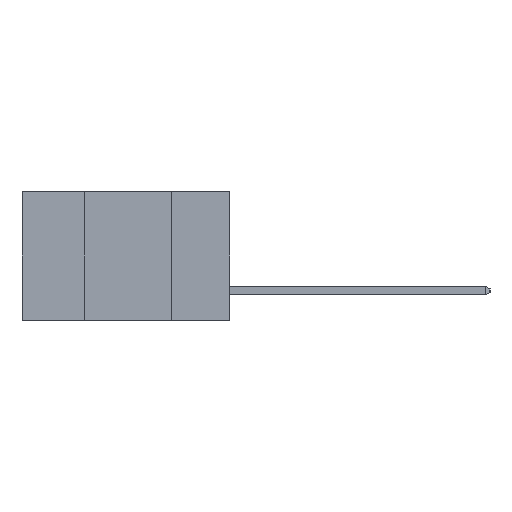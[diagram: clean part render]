
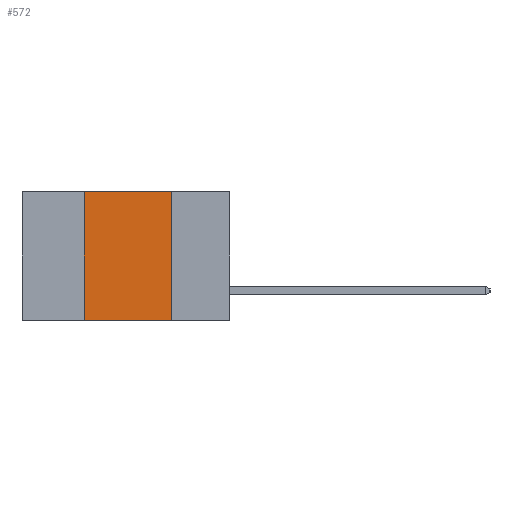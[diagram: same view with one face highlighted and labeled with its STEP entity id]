
A CAD part, left-side view. The second image highlights one B-rep face of the part: STEP entity #572.
In plain terms, the highlighted planar face has unit normal (-1, 0, 0).
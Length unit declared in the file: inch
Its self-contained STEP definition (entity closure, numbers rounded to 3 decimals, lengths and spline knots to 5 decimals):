
#27 = VECTOR ( 'NONE', #4501, 39.37008 ) ;
#572 = ADVANCED_FACE ( 'NONE', ( #13866 ), #2486, .F. ) ;
#588 = CARTESIAN_POINT ( 'NONE',  ( 0., 0.17, -0.37 ) ) ;
#597 = VECTOR ( 'NONE', #9261, 39.37008 ) ;
#619 = EDGE_CURVE ( 'NONE', #12613, #11998, #4045, .T. ) ;
#2079 = EDGE_CURVE ( 'NONE', #2499, #9808, #2431, .T. ) ;
#2112 = CARTESIAN_POINT ( 'NONE',  ( 0., 0.42, 0. ) ) ;
#2414 = EDGE_CURVE ( 'NONE', #12613, #2499, #10024, .T. ) ;
#2431 = LINE ( 'NONE', #4407, #27 ) ;
#2486 = PLANE ( 'NONE',  #6173 ) ;
#2499 = VERTEX_POINT ( 'NONE', #2112 ) ;
#2642 = CARTESIAN_POINT ( 'NONE',  ( 0., 0.17, -0.37 ) ) ;
#3375 = ORIENTED_EDGE ( 'NONE', *, *, #2414, .F. ) ;
#4045 = LINE ( 'NONE', #12520, #4383 ) ;
#4383 = VECTOR ( 'NONE', #11346, 39.37008 ) ;
#4407 = CARTESIAN_POINT ( 'NONE',  ( 0., 0.6, 0. ) ) ;
#4501 = DIRECTION ( 'NONE',  ( 0., -1., 0. ) ) ;
#6173 = AXIS2_PLACEMENT_3D ( 'NONE', #8083, #8129, #6922 ) ;
#6922 = DIRECTION ( 'NONE',  ( 0., 0., -1. ) ) ;
#6966 = CARTESIAN_POINT ( 'NONE',  ( 0., 0.42, -0.37 ) ) ;
#7098 = VECTOR ( 'NONE', #12920, 39.37008 ) ;
#7394 = CARTESIAN_POINT ( 'NONE',  ( 0., 0.42, -0.37 ) ) ;
#8083 = CARTESIAN_POINT ( 'NONE',  ( 0., 0.6, 0. ) ) ;
#8129 = DIRECTION ( 'NONE',  ( 1., 0., 0. ) ) ;
#8370 = ORIENTED_EDGE ( 'NONE', *, *, #8937, .F. ) ;
#8937 = EDGE_CURVE ( 'NONE', #9808, #11998, #14173, .T. ) ;
#9261 = DIRECTION ( 'NONE',  ( 0., 0., -1. ) ) ;
#9808 = VERTEX_POINT ( 'NONE', #12614 ) ;
#10024 = LINE ( 'NONE', #7394, #7098 ) ;
#11346 = DIRECTION ( 'NONE',  ( 0., -1., 0. ) ) ;
#11998 = VERTEX_POINT ( 'NONE', #2642 ) ;
#12431 = ORIENTED_EDGE ( 'NONE', *, *, #619, .T. ) ;
#12520 = CARTESIAN_POINT ( 'NONE',  ( 0., 0.6, -0.37 ) ) ;
#12613 = VERTEX_POINT ( 'NONE', #6966 ) ;
#12614 = CARTESIAN_POINT ( 'NONE',  ( 0., 0.17, 0. ) ) ;
#12920 = DIRECTION ( 'NONE',  ( 0., 0., 1. ) ) ;
#13584 = EDGE_LOOP ( 'NONE', ( #8370, #14215, #3375, #12431 ) ) ;
#13866 = FACE_OUTER_BOUND ( 'NONE', #13584, .T. ) ;
#14173 = LINE ( 'NONE', #588, #597 ) ;
#14215 = ORIENTED_EDGE ( 'NONE', *, *, #2079, .F. ) ;
